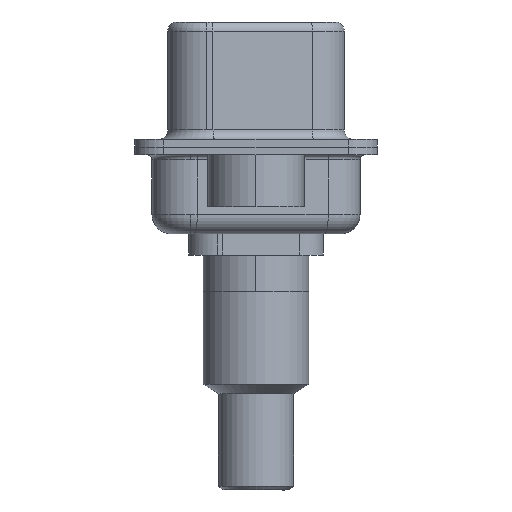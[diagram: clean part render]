
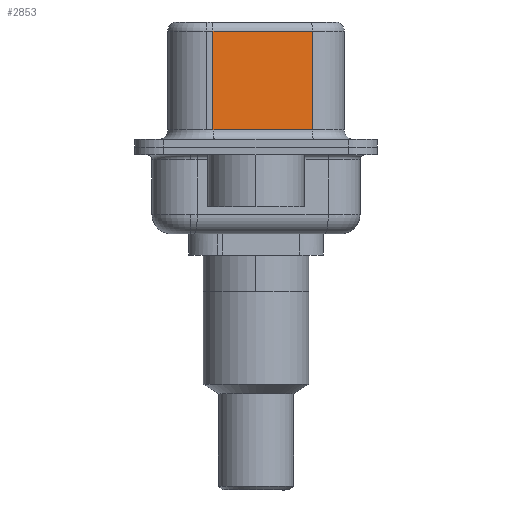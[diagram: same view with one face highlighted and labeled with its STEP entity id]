
A CAD part, left-side view. The second image highlights one B-rep face of the part: STEP entity #2853.
In plain terms, the highlighted planar face has unit normal (-0.985, -0.174, 0).
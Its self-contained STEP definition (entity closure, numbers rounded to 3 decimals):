
#673 = CARTESIAN_POINT ( 'NONE',  ( 4.565, -2.927, 6.02 ) ) ;
#1316 = VECTOR ( 'NONE', #2216, 1000. ) ;
#1361 = ORIENTED_EDGE ( 'NONE', *, *, #4673, .T. ) ;
#1954 = CARTESIAN_POINT ( 'NONE',  ( 4.565, -2.927, 0.9 ) ) ;
#2216 = DIRECTION ( 'NONE',  ( -0.174, 0.985, 0. ) ) ;
#2853 = ADVANCED_FACE ( 'NONE', ( #14151 ), #9092, .F. ) ;
#4445 = EDGE_LOOP ( 'NONE', ( #15267, #17612, #1361, #9243 ) ) ;
#4448 = CARTESIAN_POINT ( 'NONE',  ( 3.655, 2.233, 6.02 ) ) ;
#4640 = DIRECTION ( 'NONE',  ( 0.174, -0.985, 0. ) ) ;
#4673 = EDGE_CURVE ( 'NONE', #5702, #4703, #7112, .T. ) ;
#4703 = VERTEX_POINT ( 'NONE', #16356 ) ;
#5702 = VERTEX_POINT ( 'NONE', #4448 ) ;
#6021 = EDGE_CURVE ( 'NONE', #15590, #10704, #16924, .T. ) ;
#6834 = CARTESIAN_POINT ( 'NONE',  ( 4.565, -2.927, 6.52 ) ) ;
#7112 = LINE ( 'NONE', #14506, #10529 ) ;
#7594 = AXIS2_PLACEMENT_3D ( 'NONE', #6834, #8288, #18242 ) ;
#8288 = DIRECTION ( 'NONE',  ( 0.985, 0.174, 0. ) ) ;
#9092 = PLANE ( 'NONE',  #7594 ) ;
#9243 = ORIENTED_EDGE ( 'NONE', *, *, #11254, .T. ) ;
#9558 = DIRECTION ( 'NONE',  ( 0., 0., -1. ) ) ;
#10269 = VECTOR ( 'NONE', #4640, 1000. ) ;
#10473 = CARTESIAN_POINT ( 'NONE',  ( 4.565, -2.927, 0.9 ) ) ;
#10529 = VECTOR ( 'NONE', #9558, 1000. ) ;
#10704 = VERTEX_POINT ( 'NONE', #1954 ) ;
#11254 = EDGE_CURVE ( 'NONE', #4703, #10704, #14064, .T. ) ;
#12443 = CARTESIAN_POINT ( 'NONE',  ( 4.565, -2.927, 6.02 ) ) ;
#13010 = LINE ( 'NONE', #12443, #1316 ) ;
#13094 = VECTOR ( 'NONE', #14415, 1000. ) ;
#13326 = EDGE_CURVE ( 'NONE', #15590, #5702, #13010, .T. ) ;
#14064 = LINE ( 'NONE', #10473, #10269 ) ;
#14151 = FACE_OUTER_BOUND ( 'NONE', #4445, .T. ) ;
#14415 = DIRECTION ( 'NONE',  ( 0., 0., -1. ) ) ;
#14506 = CARTESIAN_POINT ( 'NONE',  ( 3.655, 2.233, 6.52 ) ) ;
#15267 = ORIENTED_EDGE ( 'NONE', *, *, #6021, .F. ) ;
#15590 = VERTEX_POINT ( 'NONE', #673 ) ;
#16356 = CARTESIAN_POINT ( 'NONE',  ( 3.655, 2.233, 0.9 ) ) ;
#16774 = CARTESIAN_POINT ( 'NONE',  ( 4.565, -2.927, 6.52 ) ) ;
#16924 = LINE ( 'NONE', #16774, #13094 ) ;
#17612 = ORIENTED_EDGE ( 'NONE', *, *, #13326, .T. ) ;
#18242 = DIRECTION ( 'NONE',  ( -0.174, 0.985, 0. ) ) ;
